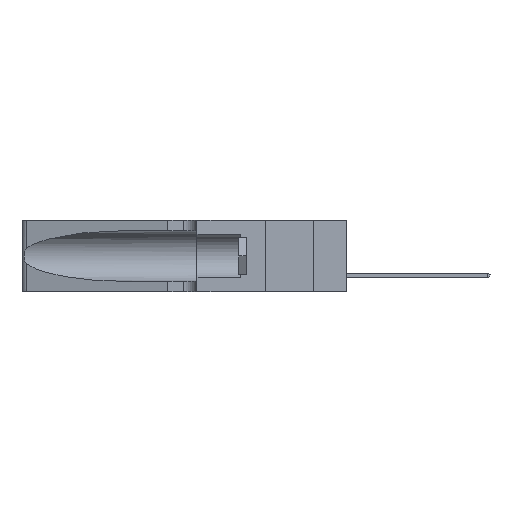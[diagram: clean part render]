
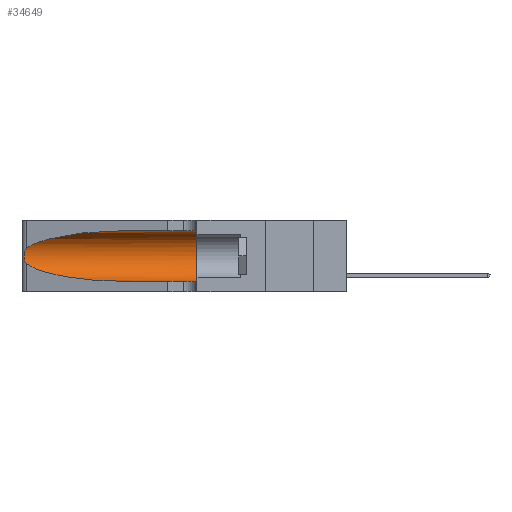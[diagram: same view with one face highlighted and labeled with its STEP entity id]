
A CAD part, left-side view. The second image highlights one B-rep face of the part: STEP entity #34649.
In plain terms, the highlighted cylindrical face has radius 3.308 mm (diameter 6.617 mm), a partial arc.
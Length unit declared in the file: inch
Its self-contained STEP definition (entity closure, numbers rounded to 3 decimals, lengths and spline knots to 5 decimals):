
#416 = VERTEX_POINT ( 'NONE', #15564 ) ;
#629 = VERTEX_POINT ( 'NONE', #39908 ) ;
#2429 = EDGE_CURVE ( 'NONE', #23783, #10067, #13519, .T. ) ;
#2749 = ORIENTED_EDGE ( 'NONE', *, *, #41438, .T. ) ;
#3423 = CARTESIAN_POINT ( 'NONE',  ( 0.25487, 1.22718, 0.22369 ) ) ;
#4146 = DIRECTION ( 'NONE',  ( 0., -1., 0. ) ) ;
#4562 = CYLINDRICAL_SURFACE ( 'NONE', #31263, 0.13025 ) ;
#5933 = CARTESIAN_POINT ( 'NONE',  ( 0.25487, 1.22718, 0.22369 ) ) ;
#6273 =( BOUNDED_CURVE ( )  B_SPLINE_CURVE ( 3, ( #41434, #20998, #11650, #35134 ),
 .UNSPECIFIED., .F., .F. ) 
 B_SPLINE_CURVE_WITH_KNOTS ( ( 4, 4 ),
 ( 1.5708, 2.84003 ),
 .UNSPECIFIED. ) 
 CURVE ( )  GEOMETRIC_REPRESENTATION_ITEM ( )  RATIONAL_B_SPLINE_CURVE ( ( 1., 0.87, 0.87, 1. ) ) 
 REPRESENTATION_ITEM ( '' )  );
#6701 = EDGE_LOOP ( 'NONE', ( #32392, #25252, #2749, #11925, #41968, #33995 ) ) ;
#7033 = CARTESIAN_POINT ( 'NONE',  ( 0.1305, 1.61858, 0.185 ) ) ;
#8864 = CARTESIAN_POINT ( 'NONE',  ( 0.1305, 0.35, 0.185 ) ) ;
#9292 = CARTESIAN_POINT ( 'NONE',  ( 0.26017, 1.23833, 0.17102 ) ) ;
#9714 = CARTESIAN_POINT ( 'NONE',  ( 0.25555, 1.22994, 0.2215 ) ) ;
#10021 = CARTESIAN_POINT ( 'NONE',  ( 0.1305, 0.72297, 0.05475 ) ) ;
#10067 = VERTEX_POINT ( 'NONE', #42522 ) ;
#10250 = DIRECTION ( 'NONE',  ( 0., 0., -1. ) ) ;
#11342 = CARTESIAN_POINT ( 'NONE',  ( 0.1305, 0.35, 0.31525 ) ) ;
#11650 = CARTESIAN_POINT ( 'NONE',  ( 0.2373, 1.15595, 0.28018 ) ) ;
#11925 = ORIENTED_EDGE ( 'NONE', *, *, #2429, .T. ) ;
#13151 = CARTESIAN_POINT ( 'NONE',  ( 0.25789, 1.23486, 0.15765 ) ) ;
#13519 = LINE ( 'NONE', #43114, #25608 ) ;
#13904 = DIRECTION ( 'NONE',  ( 0., -1., 0. ) ) ;
#14163 = VERTEX_POINT ( 'NONE', #11342 ) ;
#14470 = FACE_OUTER_BOUND ( 'NONE', #6701, .T. ) ;
#15337 = B_SPLINE_CURVE_WITH_KNOTS ( 'NONE', 3,
 ( #5933, #9714, #36495, #19486, #42828, #33023, #22822, #16386, #9292, #32884, #13151, #19766, #22538, #37790 ),
 .UNSPECIFIED., .F., .F.,
 ( 4, 2, 2, 2, 2, 2, 4 ),
 ( 0., 0.00027, 0.00053, 0.00107, 0.0016, 0.00187, 0.00214 ),
 .UNSPECIFIED. ) ;
#15564 = CARTESIAN_POINT ( 'NONE',  ( 0.25487, 1.22718, 0.14631 ) ) ;
#15853 = DIRECTION ( 'NONE',  ( 0., 1., 0. ) ) ;
#15975 = LINE ( 'NONE', #33749, #23217 ) ;
#16386 = CARTESIAN_POINT ( 'NONE',  ( 0.26075, 1.23896, 0.178 ) ) ;
#16656 = EDGE_CURVE ( 'NONE', #42654, #416, #15337, .T. ) ;
#16897 = AXIS2_PLACEMENT_3D ( 'NONE', #8864, #15853, #32349 ) ;
#17926 = EDGE_CURVE ( 'NONE', #14163, #10067, #31295, .T. ) ;
#19486 = CARTESIAN_POINT ( 'NONE',  ( 0.25787, 1.23484, 0.2124 ) ) ;
#19766 = CARTESIAN_POINT ( 'NONE',  ( 0.25639, 1.23186, 0.15144 ) ) ;
#20505 = CARTESIAN_POINT ( 'NONE',  ( 0.18966, 0.96281, 0.05475 ) ) ;
#20649 = EDGE_CURVE ( 'NONE', #629, #14163, #15975, .T. ) ;
#20998 = CARTESIAN_POINT ( 'NONE',  ( 0.18966, 0.96281, 0.31525 ) ) ;
#22538 = CARTESIAN_POINT ( 'NONE',  ( 0.25555, 1.22993, 0.14849 ) ) ;
#22822 = CARTESIAN_POINT ( 'NONE',  ( 0.26075, 1.23896, 0.19203 ) ) ;
#23217 = VECTOR ( 'NONE', #13904, 39.37008 ) ;
#23783 = VERTEX_POINT ( 'NONE', #30997 ) ;
#23967 = CARTESIAN_POINT ( 'NONE',  ( 0.2373, 1.15595, 0.08982 ) ) ;
#25252 = ORIENTED_EDGE ( 'NONE', *, *, #16656, .T. ) ;
#25608 = VECTOR ( 'NONE', #33175, 39.37008 ) ;
#30997 = CARTESIAN_POINT ( 'NONE',  ( 0.1305, 0.72297, 0.05475 ) ) ;
#31263 = AXIS2_PLACEMENT_3D ( 'NONE', #7033, #4146, #10250 ) ;
#31295 = CIRCLE ( 'NONE', #16897, 0.13025 ) ;
#32349 = DIRECTION ( 'NONE',  ( 0., 0., 1. ) ) ;
#32392 = ORIENTED_EDGE ( 'NONE', *, *, #36300, .T. ) ;
#32884 = CARTESIAN_POINT ( 'NONE',  ( 0.25856, 1.23593, 0.16098 ) ) ;
#33023 = CARTESIAN_POINT ( 'NONE',  ( 0.26018, 1.23835, 0.19895 ) ) ;
#33175 = DIRECTION ( 'NONE',  ( 0., -1., 0. ) ) ;
#33749 = CARTESIAN_POINT ( 'NONE',  ( 0.1305, 1.61858, 0.31525 ) ) ;
#33995 = ORIENTED_EDGE ( 'NONE', *, *, #20649, .F. ) ;
#34649 = ADVANCED_FACE ( 'NONE', ( #14470 ), #4562, .F. ) ;
#35134 = CARTESIAN_POINT ( 'NONE',  ( 0.25487, 1.22718, 0.22369 ) ) ;
#36300 = EDGE_CURVE ( 'NONE', #629, #42654, #6273, .T. ) ;
#36495 = CARTESIAN_POINT ( 'NONE',  ( 0.25639, 1.23184, 0.21858 ) ) ;
#37790 = CARTESIAN_POINT ( 'NONE',  ( 0.25487, 1.22718, 0.14631 ) ) ;
#39908 = CARTESIAN_POINT ( 'NONE',  ( 0.1305, 0.72297, 0.31525 ) ) ;
#40452 = CARTESIAN_POINT ( 'NONE',  ( 0.25487, 1.22718, 0.14631 ) ) ;
#41434 = CARTESIAN_POINT ( 'NONE',  ( 0.1305, 0.72297, 0.31525 ) ) ;
#41438 = EDGE_CURVE ( 'NONE', #416, #23783, #41839, .T. ) ;
#41839 =( BOUNDED_CURVE ( )  B_SPLINE_CURVE ( 3, ( #40452, #23967, #20505, #10021 ),
 .UNSPECIFIED., .F., .T. ) 
 B_SPLINE_CURVE_WITH_KNOTS ( ( 4, 4 ),
 ( 3.44316, 4.71239 ),
 .UNSPECIFIED. ) 
 CURVE ( )  GEOMETRIC_REPRESENTATION_ITEM ( )  RATIONAL_B_SPLINE_CURVE ( ( 1., 0.87, 0.87, 1. ) ) 
 REPRESENTATION_ITEM ( '' )  );
#41968 = ORIENTED_EDGE ( 'NONE', *, *, #17926, .F. ) ;
#42522 = CARTESIAN_POINT ( 'NONE',  ( 0.1305, 0.35, 0.05475 ) ) ;
#42654 = VERTEX_POINT ( 'NONE', #3423 ) ;
#42828 = CARTESIAN_POINT ( 'NONE',  ( 0.25854, 1.2359, 0.20912 ) ) ;
#43114 = CARTESIAN_POINT ( 'NONE',  ( 0.1305, 1.61858, 0.05475 ) ) ;
